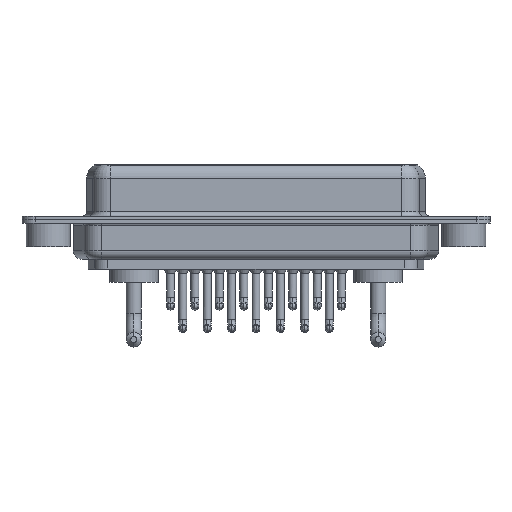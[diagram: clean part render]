
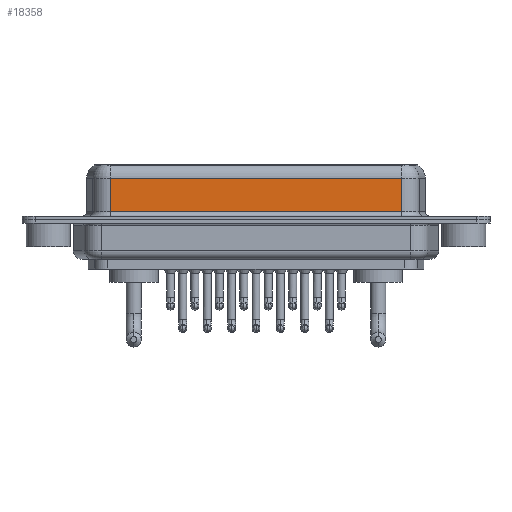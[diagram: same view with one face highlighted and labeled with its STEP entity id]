
A CAD part, front view. The second image highlights one B-rep face of the part: STEP entity #18358.
In plain terms, the highlighted planar face has unit normal (0, -1, 0).
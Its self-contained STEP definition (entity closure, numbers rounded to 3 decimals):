
#96 = ORIENTED_EDGE ( 'NONE', *, *, #11416, .T. ) ;
#909 = VECTOR ( 'NONE', #8577, 1000. ) ;
#3229 = LINE ( 'NONE', #16167, #11480 ) ;
#3728 = LINE ( 'NONE', #5205, #909 ) ;
#3944 = VECTOR ( 'NONE', #17596, 1000. ) ;
#4649 = DIRECTION ( 'NONE',  ( 0., 0., 1. ) ) ;
#5057 = EDGE_CURVE ( 'NONE', #16321, #18828, #15928, .T. ) ;
#5205 = CARTESIAN_POINT ( 'NONE',  ( 40.037, -3.95, 4.65 ) ) ;
#6350 = EDGE_CURVE ( 'NONE', #16321, #7508, #3728, .T. ) ;
#6564 = ORIENTED_EDGE ( 'NONE', *, *, #9564, .T. ) ;
#6826 = LINE ( 'NONE', #13241, #17481 ) ;
#7508 = VERTEX_POINT ( 'NONE', #14010 ) ;
#8577 = DIRECTION ( 'NONE',  ( -1., 0., 0. ) ) ;
#9201 = FACE_OUTER_BOUND ( 'NONE', #12595, .T. ) ;
#9564 = EDGE_CURVE ( 'NONE', #18830, #18828, #6826, .T. ) ;
#11193 = CARTESIAN_POINT ( 'NONE',  ( 40.037, -3.95, 6.4 ) ) ;
#11227 = DIRECTION ( 'NONE',  ( 0., 0., -1. ) ) ;
#11416 = EDGE_CURVE ( 'NONE', #7508, #18830, #3229, .T. ) ;
#11445 = DIRECTION ( 'NONE',  ( 1., 0., 0. ) ) ;
#11480 = VECTOR ( 'NONE', #11227, 1000. ) ;
#12353 = PLANE ( 'NONE',  #19209 ) ;
#12595 = EDGE_LOOP ( 'NONE', ( #17796, #13501, #96, #6564 ) ) ;
#12632 = CARTESIAN_POINT ( 'NONE',  ( 40.037, -3.95, 0.9 ) ) ;
#12734 = CARTESIAN_POINT ( 'NONE',  ( 7.013, -3.95, 0.9 ) ) ;
#12757 = DIRECTION ( 'NONE',  ( 0., 1., 0. ) ) ;
#13241 = CARTESIAN_POINT ( 'NONE',  ( 40.037, -3.95, 0.9 ) ) ;
#13501 = ORIENTED_EDGE ( 'NONE', *, *, #6350, .T. ) ;
#13856 = CARTESIAN_POINT ( 'NONE',  ( 40.037, -3.95, 4.65 ) ) ;
#14010 = CARTESIAN_POINT ( 'NONE',  ( 7.013, -3.95, 4.65 ) ) ;
#15928 = LINE ( 'NONE', #11193, #3944 ) ;
#16167 = CARTESIAN_POINT ( 'NONE',  ( 7.013, -3.95, 6.4 ) ) ;
#16321 = VERTEX_POINT ( 'NONE', #13856 ) ;
#17481 = VECTOR ( 'NONE', #11445, 1000. ) ;
#17596 = DIRECTION ( 'NONE',  ( 0., 0., -1. ) ) ;
#17796 = ORIENTED_EDGE ( 'NONE', *, *, #5057, .F. ) ;
#18358 = ADVANCED_FACE ( 'NONE', ( #9201 ), #12353, .F. ) ;
#18828 = VERTEX_POINT ( 'NONE', #12632 ) ;
#18830 = VERTEX_POINT ( 'NONE', #12734 ) ;
#19074 = CARTESIAN_POINT ( 'NONE',  ( 40.037, -3.95, 6.4 ) ) ;
#19209 = AXIS2_PLACEMENT_3D ( 'NONE', #19074, #12757, #4649 ) ;
